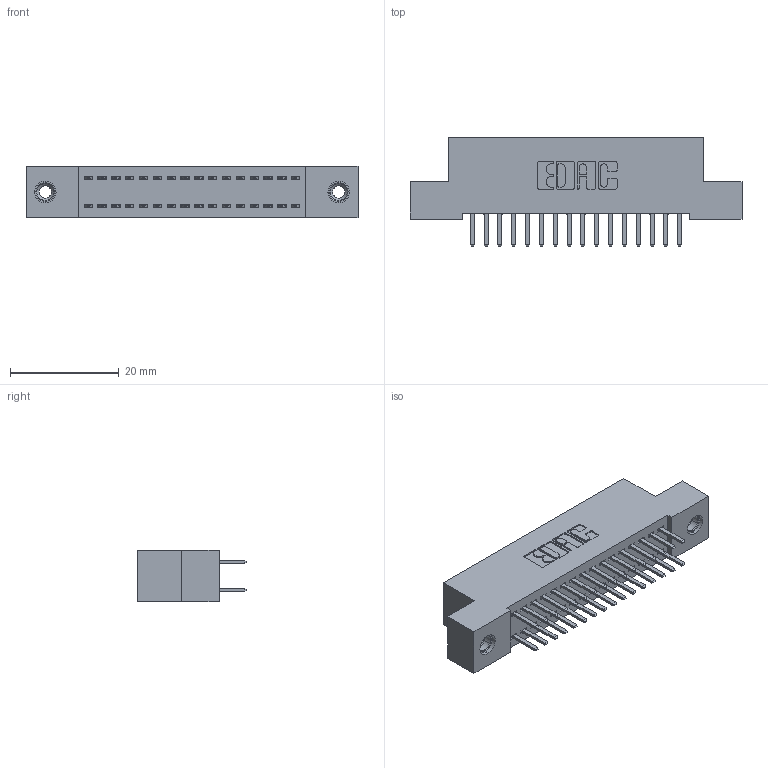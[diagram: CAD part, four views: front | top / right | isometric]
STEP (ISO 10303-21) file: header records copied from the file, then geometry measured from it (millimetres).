
FILE_DESCRIPTION (( 'STEP AP203' ), '1' );
FILE_NAME ('392-032-520-208.STEP', '2019-10-07T14:20:02', ( '' ), ( '' ), 'SwSTEP 2.0', 'SolidWorks 2016', '' );
FILE_SCHEMA (( 'CONFIG_CONTROL_DESIGN' ));
Length unit declared in the file: inch
Products named in the file (4): 342 Part_TI; 345-292-001_345-293-120; 345-250-001_345-250-003-102; 392-032-520-208
Assembly tree (35 placements, depth 2):
  392-032-520-208
    342 Part_TI
    345-292-001_345-293-120  x32
    345-250-001_345-250-003-102  x2
Bounding box: 60.96 x 20.02 x 9.4 mm (x, y, z)
Volume: 5334.4 mm3; surface area: 8019.5 mm2
Topology: 35 solids, 35 shells, 1962 faces, 5651 edges, 3674 vertices
Faces by surface type: plane 1314, cylinder 632, cone 12, torus 4
Entity records: 14824 total; most frequent: CARTESIAN_POINT 2481, ORIENTED_EDGE 2398, DIRECTION 2185, EDGE_CURVE 1199, VECTOR 1047, LINE 1047, VERTEX_POINT 792, AXIS2_PLACEMENT_3D 569
